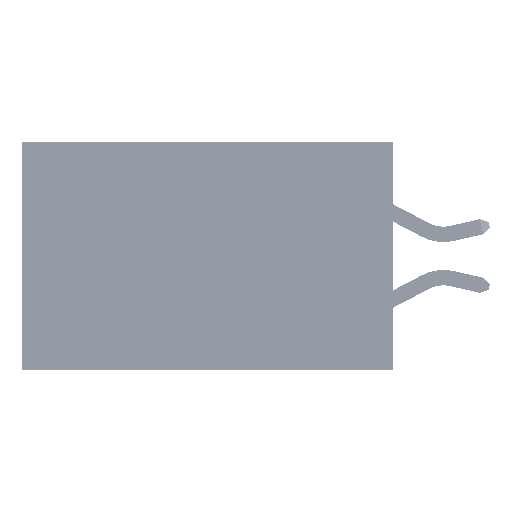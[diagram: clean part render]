
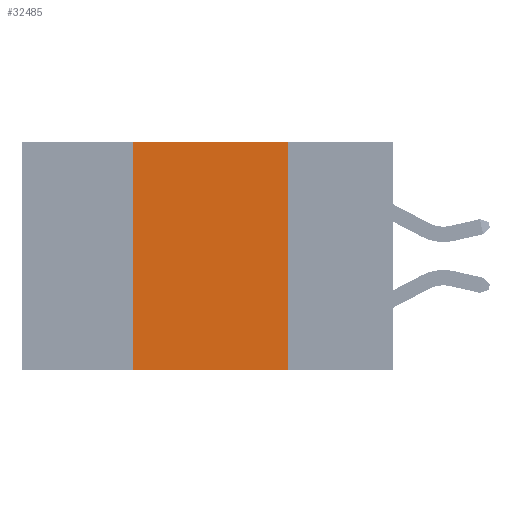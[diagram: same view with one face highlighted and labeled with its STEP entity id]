
A CAD part, left-side view. The second image highlights one B-rep face of the part: STEP entity #32485.
In plain terms, the highlighted planar face has unit normal (-1, 0, 0).
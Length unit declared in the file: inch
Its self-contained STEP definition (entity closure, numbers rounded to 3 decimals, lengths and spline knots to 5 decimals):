
#1224 = ORIENTED_EDGE ( 'NONE', *, *, #16918, .F. ) ;
#1453 = LINE ( 'NONE', #3155, #15810 ) ;
#2411 = EDGE_CURVE ( 'NONE', #2641, #45064, #21525, .T. ) ;
#2582 = CARTESIAN_POINT ( 'NONE',  ( 0., 0.6, 0. ) ) ;
#2641 = VERTEX_POINT ( 'NONE', #6956 ) ;
#3109 = CARTESIAN_POINT ( 'NONE',  ( 0., 0.42, 0. ) ) ;
#3155 = CARTESIAN_POINT ( 'NONE',  ( 0., 0.6, 0. ) ) ;
#5061 = EDGE_CURVE ( 'NONE', #26858, #40387, #15987, .T. ) ;
#5545 = DIRECTION ( 'NONE',  ( 1., 0., 0. ) ) ;
#6737 = VECTOR ( 'NONE', #33611, 39.37008 ) ;
#6956 = CARTESIAN_POINT ( 'NONE',  ( 0., 0.42, -0.37 ) ) ;
#9311 = CARTESIAN_POINT ( 'NONE',  ( 0., 0.17, 0. ) ) ;
#9403 = AXIS2_PLACEMENT_3D ( 'NONE', #2582, #5545, #20028 ) ;
#9557 = PLANE ( 'NONE',  #9403 ) ;
#10260 = DIRECTION ( 'NONE',  ( 0., -1., 0. ) ) ;
#15800 = ORIENTED_EDGE ( 'NONE', *, *, #25334, .T. ) ;
#15810 = VECTOR ( 'NONE', #10260, 39.37008 ) ;
#15987 = LINE ( 'NONE', #16103, #29243 ) ;
#16103 = CARTESIAN_POINT ( 'NONE',  ( 0., 0.17, 0. ) ) ;
#16918 = EDGE_CURVE ( 'NONE', #45064, #26858, #1453, .T. ) ;
#19486 = DIRECTION ( 'NONE',  ( 0., 0., -1. ) ) ;
#20028 = DIRECTION ( 'NONE',  ( 0., 0., -1. ) ) ;
#21525 = LINE ( 'NONE', #3109, #32588 ) ;
#24069 = ORIENTED_EDGE ( 'NONE', *, *, #5061, .F. ) ;
#25334 = EDGE_CURVE ( 'NONE', #2641, #40387, #41944, .T. ) ;
#26858 = VERTEX_POINT ( 'NONE', #9311 ) ;
#29243 = VECTOR ( 'NONE', #19486, 39.37008 ) ;
#30457 = CARTESIAN_POINT ( 'NONE',  ( 0., 0.17, -0.37 ) ) ;
#31971 = ORIENTED_EDGE ( 'NONE', *, *, #2411, .F. ) ;
#32485 = ADVANCED_FACE ( 'NONE', ( #42342 ), #9557, .F. ) ;
#32588 = VECTOR ( 'NONE', #41555, 39.37008 ) ;
#33611 = DIRECTION ( 'NONE',  ( 0., -1., 0. ) ) ;
#33768 = CARTESIAN_POINT ( 'NONE',  ( 0., 0.6, -0.37 ) ) ;
#39617 = CARTESIAN_POINT ( 'NONE',  ( 0., 0.42, 0. ) ) ;
#40387 = VERTEX_POINT ( 'NONE', #30457 ) ;
#41555 = DIRECTION ( 'NONE',  ( 0., 0., 1. ) ) ;
#41944 = LINE ( 'NONE', #33768, #6737 ) ;
#42342 = FACE_OUTER_BOUND ( 'NONE', #43131, .T. ) ;
#43131 = EDGE_LOOP ( 'NONE', ( #24069, #1224, #31971, #15800 ) ) ;
#45064 = VERTEX_POINT ( 'NONE', #39617 ) ;
